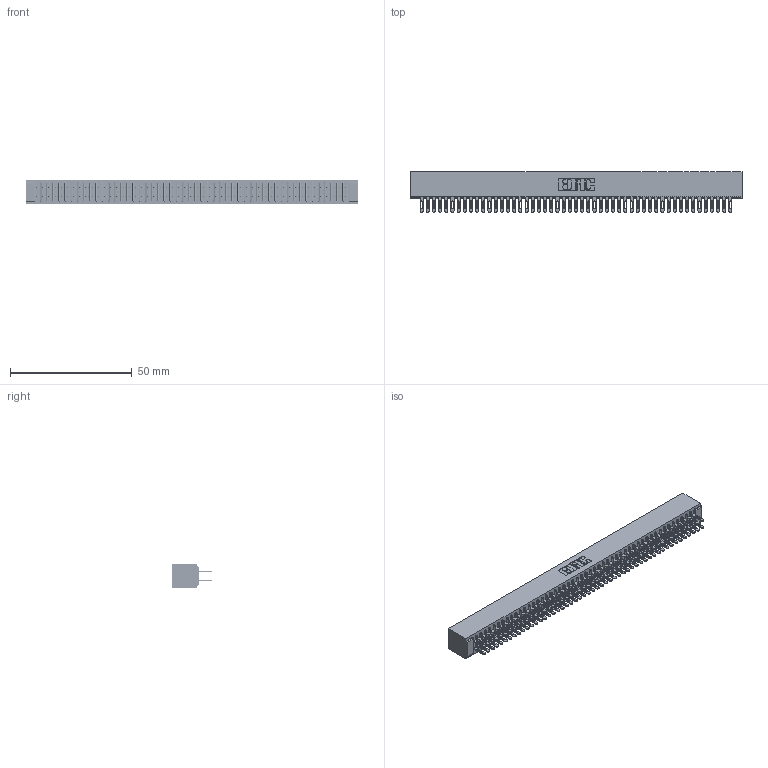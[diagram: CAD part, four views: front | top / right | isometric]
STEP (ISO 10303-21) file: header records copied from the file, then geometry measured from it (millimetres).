
FILE_DESCRIPTION (( 'STEP AP203' ), '1' );
FILE_NAME ('341-102-500-201.STEP', '2018-08-08T03:08:11', ( '' ), ( '' ), 'SwSTEP 2.0', 'SolidWorks 2016', '' );
FILE_SCHEMA (( 'CONFIG_CONTROL_DESIGN' ));
Length unit declared in the file: inch
Products named in the file (3): 341 Part_No Mounting Lugs; 341-292-001_341-292-100; 341-102-500-201
Assembly tree (103 placements, depth 2):
  341-102-500-201
    341 Part_No Mounting Lugs
    341-292-001_341-292-100  x102
Bounding box: 136.53 x 16.69 x 10.16 mm (x, y, z)
Volume: 10457.2 mm3; surface area: 20359.7 mm2
Topology: 103 solids, 103 shells, 6840 faces, 19825 edges, 12838 vertices
Faces by surface type: plane 3940, cylinder 2696, sphere 104, torus 100
Entity records: 60252 total; most frequent: CARTESIAN_POINT 10013, ORIENTED_EDGE 9950, DIRECTION 9713, EDGE_CURVE 4975, VECTOR 4029, LINE 4029, VERTEX_POINT 3142, AXIS2_PLACEMENT_3D 2842
